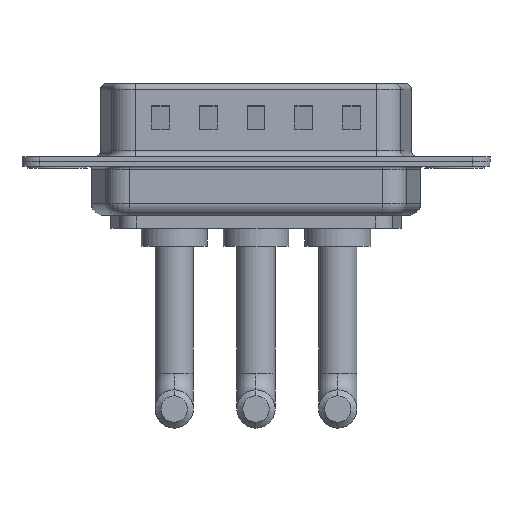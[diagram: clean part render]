
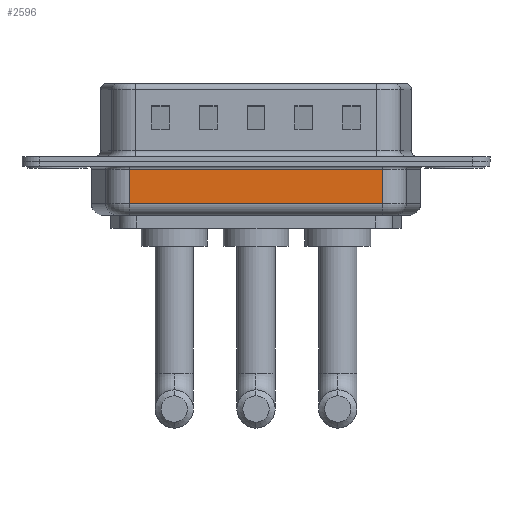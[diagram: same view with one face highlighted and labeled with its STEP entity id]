
A CAD part, front view. The second image highlights one B-rep face of the part: STEP entity #2596.
In plain terms, the highlighted planar face has unit normal (0, -1, 0).
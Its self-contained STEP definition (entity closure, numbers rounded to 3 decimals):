
#237 = CARTESIAN_POINT ( 'NONE',  ( 6.031, -5.35, -3.5 ) ) ;
#526 = PLANE ( 'NONE',  #8087 ) ;
#586 = LINE ( 'NONE', #6873, #3038 ) ;
#955 = ORIENTED_EDGE ( 'NONE', *, *, #12075, .T. ) ;
#1660 = DIRECTION ( 'NONE',  ( 0., 0., 1. ) ) ;
#1802 = CARTESIAN_POINT ( 'NONE',  ( 6.031, -5.35, -4.5 ) ) ;
#2474 = LINE ( 'NONE', #3543, #8834 ) ;
#2596 = ADVANCED_FACE ( 'NONE', ( #10099 ), #526, .F. ) ;
#2928 = VERTEX_POINT ( 'NONE', #9490 ) ;
#3038 = VECTOR ( 'NONE', #13449, 1000. ) ;
#3094 = ORIENTED_EDGE ( 'NONE', *, *, #12304, .T. ) ;
#3543 = CARTESIAN_POINT ( 'NONE',  ( 6.031, -5.35, -4.5 ) ) ;
#4071 = ORIENTED_EDGE ( 'NONE', *, *, #5390, .F. ) ;
#4536 = DIRECTION ( 'NONE',  ( 1., 0., 0. ) ) ;
#5390 = EDGE_CURVE ( 'NONE', #2928, #6860, #2474, .T. ) ;
#5511 = VERTEX_POINT ( 'NONE', #6235 ) ;
#5570 = VECTOR ( 'NONE', #4536, 1000. ) ;
#5960 = DIRECTION ( 'NONE',  ( 0., 0., 1. ) ) ;
#6019 = VERTEX_POINT ( 'NONE', #11602 ) ;
#6235 = CARTESIAN_POINT ( 'NONE',  ( 27.269, -5.35, -3.5 ) ) ;
#6269 = ORIENTED_EDGE ( 'NONE', *, *, #6572, .T. ) ;
#6306 = CARTESIAN_POINT ( 'NONE',  ( 6.031, -5.35, -0.65 ) ) ;
#6572 = EDGE_CURVE ( 'NONE', #2928, #5511, #11772, .T. ) ;
#6714 = CARTESIAN_POINT ( 'NONE',  ( 6.031, -5.35, -0.65 ) ) ;
#6860 = VERTEX_POINT ( 'NONE', #6306 ) ;
#6873 = CARTESIAN_POINT ( 'NONE',  ( 27.269, -5.35, -4.5 ) ) ;
#7093 = DIRECTION ( 'NONE',  ( 0., 1., 0. ) ) ;
#8087 = AXIS2_PLACEMENT_3D ( 'NONE', #1802, #7093, #1660 ) ;
#8235 = EDGE_LOOP ( 'NONE', ( #4071, #6269, #955, #3094 ) ) ;
#8834 = VECTOR ( 'NONE', #5960, 1000. ) ;
#9490 = CARTESIAN_POINT ( 'NONE',  ( 6.031, -5.35, -3.5 ) ) ;
#10099 = FACE_OUTER_BOUND ( 'NONE', #8235, .T. ) ;
#10770 = DIRECTION ( 'NONE',  ( -1., 0., 0. ) ) ;
#11042 = LINE ( 'NONE', #6714, #12681 ) ;
#11602 = CARTESIAN_POINT ( 'NONE',  ( 27.269, -5.35, -0.65 ) ) ;
#11772 = LINE ( 'NONE', #237, #5570 ) ;
#12075 = EDGE_CURVE ( 'NONE', #5511, #6019, #586, .T. ) ;
#12304 = EDGE_CURVE ( 'NONE', #6019, #6860, #11042, .T. ) ;
#12681 = VECTOR ( 'NONE', #10770, 1000. ) ;
#13449 = DIRECTION ( 'NONE',  ( 0., 0., 1. ) ) ;
